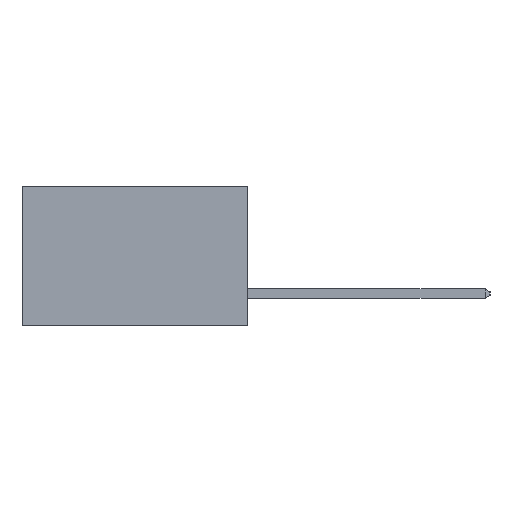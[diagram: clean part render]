
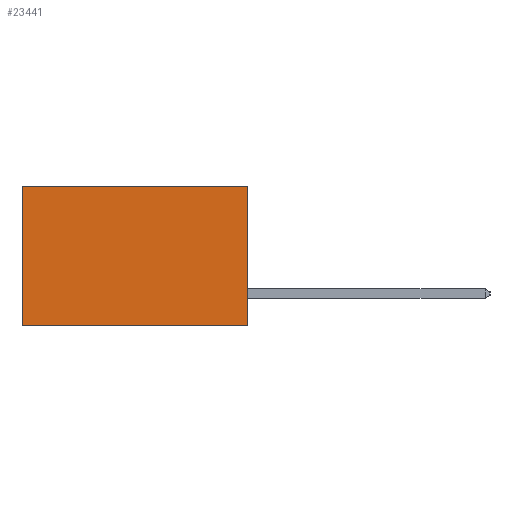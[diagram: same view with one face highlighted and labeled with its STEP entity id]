
A CAD part, left-side view. The second image highlights one B-rep face of the part: STEP entity #23441.
In plain terms, the highlighted planar face has unit normal (-1, 0, 0).
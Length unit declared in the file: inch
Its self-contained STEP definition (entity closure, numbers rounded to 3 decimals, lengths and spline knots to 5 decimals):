
#156 = PLANE ( 'NONE',  #8466 ) ;
#247 = LINE ( 'NONE', #2220, #9444 ) ;
#871 = CARTESIAN_POINT ( 'NONE',  ( 0.298, 0., 0. ) ) ;
#1025 = ORIENTED_EDGE ( 'NONE', *, *, #9552, .T. ) ;
#1857 = VERTEX_POINT ( 'NONE', #9221 ) ;
#2018 = FACE_OUTER_BOUND ( 'NONE', #4030, .T. ) ;
#2220 = CARTESIAN_POINT ( 'NONE',  ( 0.298, 0., 0. ) ) ;
#2459 = VECTOR ( 'NONE', #11333, 39.37008 ) ;
#2734 = VECTOR ( 'NONE', #2834, 39.37008 ) ;
#2834 = DIRECTION ( 'NONE',  ( 0., 0., -1. ) ) ;
#3214 = ORIENTED_EDGE ( 'NONE', *, *, #13289, .F. ) ;
#4030 = EDGE_LOOP ( 'NONE', ( #7674, #21175, #3214, #1025 ) ) ;
#6774 = CARTESIAN_POINT ( 'NONE',  ( 0.298, 0., -0.37 ) ) ;
#7116 = VERTEX_POINT ( 'NONE', #23694 ) ;
#7674 = ORIENTED_EDGE ( 'NONE', *, *, #21191, .T. ) ;
#7965 = VECTOR ( 'NONE', #18372, 39.37008 ) ;
#8004 = DIRECTION ( 'NONE',  ( 1., 0., 0. ) ) ;
#8422 = VERTEX_POINT ( 'NONE', #8694 ) ;
#8466 = AXIS2_PLACEMENT_3D ( 'NONE', #17629, #8004, #21377 ) ;
#8694 = CARTESIAN_POINT ( 'NONE',  ( 0.298, 0., 0. ) ) ;
#9221 = CARTESIAN_POINT ( 'NONE',  ( 0.298, 0.6, -0.37 ) ) ;
#9391 = CARTESIAN_POINT ( 'NONE',  ( 0.298, 0.6, 0. ) ) ;
#9444 = VECTOR ( 'NONE', #23290, 39.37008 ) ;
#9552 = EDGE_CURVE ( 'NONE', #8422, #7116, #247, .T. ) ;
#9924 = VERTEX_POINT ( 'NONE', #24319 ) ;
#11333 = DIRECTION ( 'NONE',  ( 0., 0., -1. ) ) ;
#13191 = LINE ( 'NONE', #6774, #7965 ) ;
#13289 = EDGE_CURVE ( 'NONE', #8422, #9924, #18186, .T. ) ;
#17629 = CARTESIAN_POINT ( 'NONE',  ( 0.298, 0., 0. ) ) ;
#18186 = LINE ( 'NONE', #871, #2734 ) ;
#18372 = DIRECTION ( 'NONE',  ( 0., 1., 0. ) ) ;
#21016 = EDGE_CURVE ( 'NONE', #9924, #1857, #13191, .T. ) ;
#21175 = ORIENTED_EDGE ( 'NONE', *, *, #21016, .F. ) ;
#21191 = EDGE_CURVE ( 'NONE', #7116, #1857, #22894, .T. ) ;
#21377 = DIRECTION ( 'NONE',  ( 0., 0., -1. ) ) ;
#22894 = LINE ( 'NONE', #9391, #2459 ) ;
#23290 = DIRECTION ( 'NONE',  ( 0., 1., 0. ) ) ;
#23441 = ADVANCED_FACE ( 'NONE', ( #2018 ), #156, .F. ) ;
#23694 = CARTESIAN_POINT ( 'NONE',  ( 0.298, 0.6, 0. ) ) ;
#24319 = CARTESIAN_POINT ( 'NONE',  ( 0.298, 0., -0.37 ) ) ;
